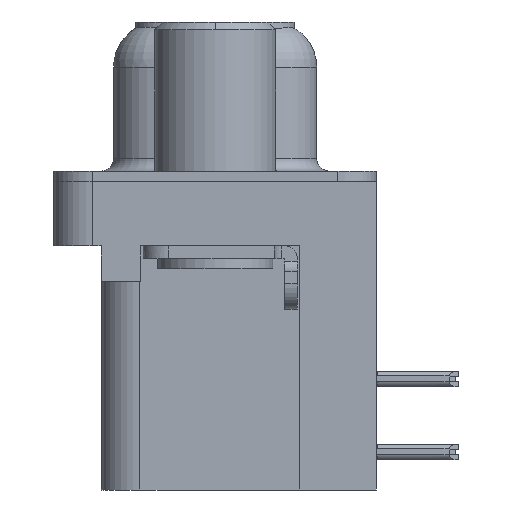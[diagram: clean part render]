
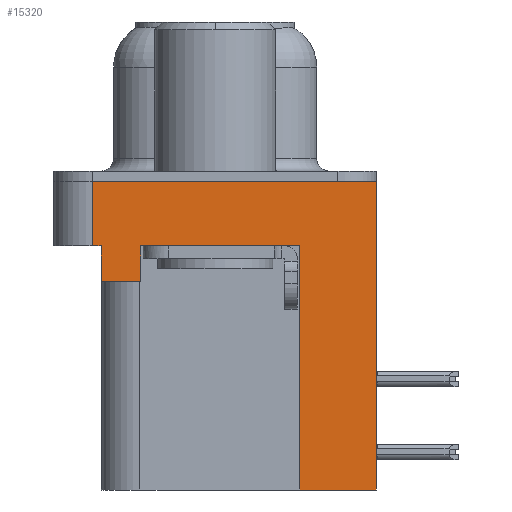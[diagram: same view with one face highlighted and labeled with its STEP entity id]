
A CAD part, left-side view. The second image highlights one B-rep face of the part: STEP entity #15320.
In plain terms, the highlighted planar face has unit normal (-1, 0, 0).
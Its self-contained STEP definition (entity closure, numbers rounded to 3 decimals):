
#508 = EDGE_CURVE ( 'NONE', #21286, #13529, #17858, .T. ) ;
#897 = CARTESIAN_POINT ( 'NONE',  ( -2.935, -6.275, -2.5 ) ) ;
#1162 = CARTESIAN_POINT ( 'NONE',  ( -2.935, 4.425, -3.9 ) ) ;
#1274 = VERTEX_POINT ( 'NONE', #11349 ) ;
#1385 = CARTESIAN_POINT ( 'NONE',  ( -2.935, 2.895, -2.5 ) ) ;
#1464 = CARTESIAN_POINT ( 'NONE',  ( -2.935, 4.425, -3.9 ) ) ;
#2119 = VECTOR ( 'NONE', #18824, 1000. ) ;
#2826 = VECTOR ( 'NONE', #23520, 1000. ) ;
#3026 = ORIENTED_EDGE ( 'NONE', *, *, #20485, .T. ) ;
#3230 = LINE ( 'NONE', #18116, #14152 ) ;
#3640 = EDGE_CURVE ( 'NONE', #13428, #13529, #22556, .T. ) ;
#3752 = DIRECTION ( 'NONE',  ( 0., 0., 1. ) ) ;
#3772 = DIRECTION ( 'NONE',  ( 0., 0., 1. ) ) ;
#5497 = DIRECTION ( 'NONE',  ( 0., 1., 0. ) ) ;
#5545 = PLANE ( 'NONE',  #25561 ) ;
#5956 = ORIENTED_EDGE ( 'NONE', *, *, #16644, .F. ) ;
#6009 = LINE ( 'NONE', #22177, #21122 ) ;
#6080 = DIRECTION ( 'NONE',  ( 0., 1., 0. ) ) ;
#6346 = VERTEX_POINT ( 'NONE', #18061 ) ;
#6744 = CARTESIAN_POINT ( 'NONE',  ( -2.935, 2.895, -3.9 ) ) ;
#6877 = DIRECTION ( 'NONE',  ( 0., 0., 1. ) ) ;
#7060 = ORIENTED_EDGE ( 'NONE', *, *, #11556, .T. ) ;
#7336 = CARTESIAN_POINT ( 'NONE',  ( -2.935, 4.775, 0. ) ) ;
#7661 = EDGE_CURVE ( 'NONE', #6346, #23163, #8273, .T. ) ;
#7715 = VERTEX_POINT ( 'NONE', #1162 ) ;
#8032 = VERTEX_POINT ( 'NONE', #7336 ) ;
#8189 = CARTESIAN_POINT ( 'NONE',  ( -2.935, 2.895, -3.9 ) ) ;
#8273 = LINE ( 'NONE', #897, #2826 ) ;
#8334 = CARTESIAN_POINT ( 'NONE',  ( -2.935, -6.275, 0. ) ) ;
#8423 = LINE ( 'NONE', #20448, #14547 ) ;
#8991 = VERTEX_POINT ( 'NONE', #8334 ) ;
#9658 = DIRECTION ( 'NONE',  ( 0., 0., 1. ) ) ;
#10367 = LINE ( 'NONE', #22804, #20681 ) ;
#10469 = CARTESIAN_POINT ( 'NONE',  ( -2.935, -6.275, -2.5 ) ) ;
#10709 = CARTESIAN_POINT ( 'NONE',  ( -2.935, 4.425, -3.9 ) ) ;
#11349 = CARTESIAN_POINT ( 'NONE',  ( -2.935, -6.275, -12. ) ) ;
#11444 = DIRECTION ( 'NONE',  ( 0., -1., 0. ) ) ;
#11556 = EDGE_CURVE ( 'NONE', #20149, #13428, #11633, .T. ) ;
#11633 = LINE ( 'NONE', #8189, #21294 ) ;
#11864 = CARTESIAN_POINT ( 'NONE',  ( -2.935, 4.425, -2.5 ) ) ;
#13214 = ORIENTED_EDGE ( 'NONE', *, *, #3640, .T. ) ;
#13428 = VERTEX_POINT ( 'NONE', #1385 ) ;
#13451 = EDGE_CURVE ( 'NONE', #20149, #7715, #19221, .T. ) ;
#13529 = VERTEX_POINT ( 'NONE', #18068 ) ;
#14152 = VECTOR ( 'NONE', #3752, 1000. ) ;
#14547 = VECTOR ( 'NONE', #6080, 1000. ) ;
#14688 = CARTESIAN_POINT ( 'NONE',  ( -2.935, -3.295, -12. ) ) ;
#14782 = VECTOR ( 'NONE', #6877, 1000. ) ;
#15256 = ORIENTED_EDGE ( 'NONE', *, *, #18934, .F. ) ;
#15320 = ADVANCED_FACE ( 'NONE', ( #23958 ), #5545, .T. ) ;
#16116 = ORIENTED_EDGE ( 'NONE', *, *, #508, .F. ) ;
#16644 = EDGE_CURVE ( 'NONE', #8032, #8991, #10367, .T. ) ;
#17095 = ORIENTED_EDGE ( 'NONE', *, *, #25027, .F. ) ;
#17103 = VECTOR ( 'NONE', #11444, 1000. ) ;
#17858 = LINE ( 'NONE', #14688, #2119 ) ;
#18061 = CARTESIAN_POINT ( 'NONE',  ( -2.935, 4.775, -2.5 ) ) ;
#18068 = CARTESIAN_POINT ( 'NONE',  ( -2.935, -3.295, -2.5 ) ) ;
#18116 = CARTESIAN_POINT ( 'NONE',  ( -2.935, -6.275, -2.5 ) ) ;
#18382 = ORIENTED_EDGE ( 'NONE', *, *, #7661, .T. ) ;
#18824 = DIRECTION ( 'NONE',  ( 0., 0., 1. ) ) ;
#18934 = EDGE_CURVE ( 'NONE', #1274, #21286, #8423, .T. ) ;
#19221 = LINE ( 'NONE', #1464, #24680 ) ;
#19932 = CARTESIAN_POINT ( 'NONE',  ( -2.935, -6.275, -2.5 ) ) ;
#20149 = VERTEX_POINT ( 'NONE', #6744 ) ;
#20230 = LINE ( 'NONE', #10709, #14782 ) ;
#20448 = CARTESIAN_POINT ( 'NONE',  ( -2.935, -3.295, -12. ) ) ;
#20485 = EDGE_CURVE ( 'NONE', #1274, #8991, #3230, .T. ) ;
#20681 = VECTOR ( 'NONE', #24864, 1000. ) ;
#20785 = CARTESIAN_POINT ( 'NONE',  ( -2.935, -3.295, -12. ) ) ;
#21122 = VECTOR ( 'NONE', #3772, 1000. ) ;
#21286 = VERTEX_POINT ( 'NONE', #20785 ) ;
#21294 = VECTOR ( 'NONE', #22559, 1000. ) ;
#21904 = EDGE_LOOP ( 'NONE', ( #5956, #17095, #18382, #24796, #24464, #7060, #13214, #16116, #15256, #3026 ) ) ;
#21981 = DIRECTION ( 'NONE',  ( -1., 0., 0. ) ) ;
#22177 = CARTESIAN_POINT ( 'NONE',  ( -2.935, 4.775, -2.5 ) ) ;
#22556 = LINE ( 'NONE', #10469, #17103 ) ;
#22559 = DIRECTION ( 'NONE',  ( 0., 0., 1. ) ) ;
#22804 = CARTESIAN_POINT ( 'NONE',  ( -2.935, -6.275, 0. ) ) ;
#22846 = EDGE_CURVE ( 'NONE', #7715, #23163, #20230, .T. ) ;
#23163 = VERTEX_POINT ( 'NONE', #11864 ) ;
#23520 = DIRECTION ( 'NONE',  ( 0., -1., 0. ) ) ;
#23958 = FACE_OUTER_BOUND ( 'NONE', #21904, .T. ) ;
#24464 = ORIENTED_EDGE ( 'NONE', *, *, #13451, .F. ) ;
#24680 = VECTOR ( 'NONE', #5497, 1000. ) ;
#24796 = ORIENTED_EDGE ( 'NONE', *, *, #22846, .F. ) ;
#24864 = DIRECTION ( 'NONE',  ( 0., -1., 0. ) ) ;
#25027 = EDGE_CURVE ( 'NONE', #6346, #8032, #6009, .T. ) ;
#25561 = AXIS2_PLACEMENT_3D ( 'NONE', #19932, #21981, #9658 ) ;
